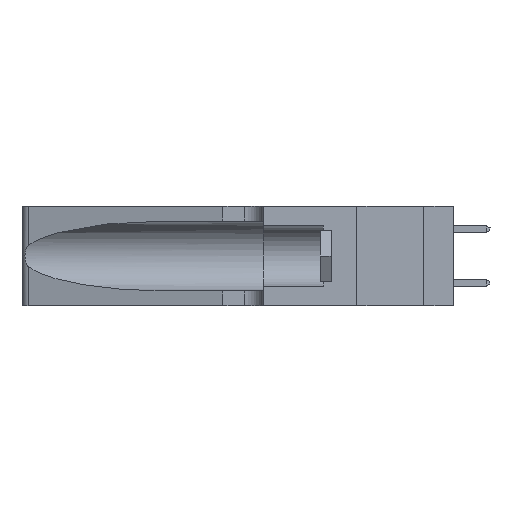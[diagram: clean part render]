
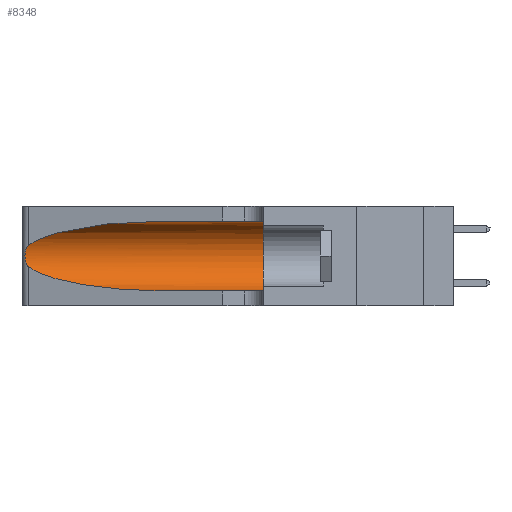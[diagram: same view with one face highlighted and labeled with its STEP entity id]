
A CAD part, left-side view. The second image highlights one B-rep face of the part: STEP entity #8348.
In plain terms, the highlighted cylindrical face has radius 3.308 mm (diameter 6.617 mm), a partial arc.
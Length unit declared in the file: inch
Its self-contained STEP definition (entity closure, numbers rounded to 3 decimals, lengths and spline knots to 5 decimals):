
#110 = VERTEX_POINT ( 'NONE', #4320 ) ;
#845 = CARTESIAN_POINT ( 'NONE',  ( 0.25856, 1.23593, 0.16098 ) ) ;
#872 = B_SPLINE_CURVE_WITH_KNOTS ( 'NONE', 3,
 ( #3177, #21387, #20005, #21594, #1643, #16368, #1378, #8098, #9783, #845, #14072, #4540, #2600, #9413 ),
 .UNSPECIFIED., .F., .F.,
 ( 4, 2, 2, 2, 2, 2, 4 ),
 ( 0., 0.00027, 0.00053, 0.00107, 0.0016, 0.00187, 0.00214 ),
 .UNSPECIFIED. ) ;
#1095 = EDGE_CURVE ( 'NONE', #14580, #16462, #4700, .T. ) ;
#1199 = CARTESIAN_POINT ( 'NONE',  ( 0.1305, 0.72297, 0.31525 ) ) ;
#1378 = CARTESIAN_POINT ( 'NONE',  ( 0.26075, 1.23896, 0.19203 ) ) ;
#1643 = CARTESIAN_POINT ( 'NONE',  ( 0.25854, 1.2359, 0.20912 ) ) ;
#1924 = CARTESIAN_POINT ( 'NONE',  ( 0.1305, 0.35, 0.185 ) ) ;
#2600 = CARTESIAN_POINT ( 'NONE',  ( 0.25555, 1.22993, 0.14849 ) ) ;
#3177 = CARTESIAN_POINT ( 'NONE',  ( 0.25487, 1.22718, 0.22369 ) ) ;
#3914 = ORIENTED_EDGE ( 'NONE', *, *, #4279, .T. ) ;
#4279 = EDGE_CURVE ( 'NONE', #16462, #14871, #872, .T. ) ;
#4320 = CARTESIAN_POINT ( 'NONE',  ( 0.1305, 0.35, 0.05475 ) ) ;
#4540 = CARTESIAN_POINT ( 'NONE',  ( 0.25639, 1.23186, 0.15144 ) ) ;
#4676 = ORIENTED_EDGE ( 'NONE', *, *, #1095, .T. ) ;
#4700 =( BOUNDED_CURVE ( )  B_SPLINE_CURVE ( 3, ( #11744, #16922, #18611, #5336 ),
 .UNSPECIFIED., .F., .T. ) 
 B_SPLINE_CURVE_WITH_KNOTS ( ( 4, 4 ),
 ( 1.5708, 2.84003 ),
 .UNSPECIFIED. ) 
 CURVE ( )  GEOMETRIC_REPRESENTATION_ITEM ( )  RATIONAL_B_SPLINE_CURVE ( ( 1., 0.87, 0.87, 1. ) ) 
 REPRESENTATION_ITEM ( '' )  );
#5022 = DIRECTION ( 'NONE',  ( 0., 1., 0. ) ) ;
#5113 = CARTESIAN_POINT ( 'NONE',  ( 0.1305, 0.72297, 0.05475 ) ) ;
#5336 = CARTESIAN_POINT ( 'NONE',  ( 0.25487, 1.22718, 0.22369 ) ) ;
#5505 = CARTESIAN_POINT ( 'NONE',  ( 0.25487, 1.22718, 0.22369 ) ) ;
#5697 = ORIENTED_EDGE ( 'NONE', *, *, #6693, .F. ) ;
#5938 = CARTESIAN_POINT ( 'NONE',  ( 0.1305, 1.61858, 0.185 ) ) ;
#6017 = VERTEX_POINT ( 'NONE', #18791 ) ;
#6693 = EDGE_CURVE ( 'NONE', #14580, #6017, #19133, .T. ) ;
#6710 = DIRECTION ( 'NONE',  ( 0., 0., 1. ) ) ;
#6713 = AXIS2_PLACEMENT_3D ( 'NONE', #1924, #5022, #6710 ) ;
#6962 =( BOUNDED_CURVE ( )  B_SPLINE_CURVE ( 3, ( #15599, #20641, #7072, #10757 ),
 .UNSPECIFIED., .F., .F. ) 
 B_SPLINE_CURVE_WITH_KNOTS ( ( 4, 4 ),
 ( 3.44316, 4.71239 ),
 .UNSPECIFIED. ) 
 CURVE ( )  GEOMETRIC_REPRESENTATION_ITEM ( )  RATIONAL_B_SPLINE_CURVE ( ( 1., 0.87, 0.87, 1. ) ) 
 REPRESENTATION_ITEM ( '' )  );
#7072 = CARTESIAN_POINT ( 'NONE',  ( 0.18966, 0.96281, 0.05475 ) ) ;
#7772 = CARTESIAN_POINT ( 'NONE',  ( 0.25487, 1.22718, 0.14631 ) ) ;
#8098 = CARTESIAN_POINT ( 'NONE',  ( 0.26075, 1.23896, 0.178 ) ) ;
#8348 = ADVANCED_FACE ( 'NONE', ( #11437 ), #17466, .F. ) ;
#8549 = VECTOR ( 'NONE', #16230, 39.37008 ) ;
#8562 = EDGE_CURVE ( 'NONE', #16965, #110, #13536, .T. ) ;
#9167 = ORIENTED_EDGE ( 'NONE', *, *, #8562, .T. ) ;
#9413 = CARTESIAN_POINT ( 'NONE',  ( 0.25487, 1.22718, 0.14631 ) ) ;
#9783 = CARTESIAN_POINT ( 'NONE',  ( 0.26017, 1.23833, 0.17102 ) ) ;
#9913 = CARTESIAN_POINT ( 'NONE',  ( 0.1305, 1.61858, 0.31525 ) ) ;
#10196 = DIRECTION ( 'NONE',  ( 0., -1., 0. ) ) ;
#10211 = VECTOR ( 'NONE', #10196, 39.37008 ) ;
#10385 = CARTESIAN_POINT ( 'NONE',  ( 0.1305, 1.61858, 0.05475 ) ) ;
#10634 = AXIS2_PLACEMENT_3D ( 'NONE', #5938, #14561, #14402 ) ;
#10757 = CARTESIAN_POINT ( 'NONE',  ( 0.1305, 0.72297, 0.05475 ) ) ;
#11437 = FACE_OUTER_BOUND ( 'NONE', #17543, .T. ) ;
#11640 = ORIENTED_EDGE ( 'NONE', *, *, #15099, .T. ) ;
#11680 = ORIENTED_EDGE ( 'NONE', *, *, #13243, .F. ) ;
#11744 = CARTESIAN_POINT ( 'NONE',  ( 0.1305, 0.72297, 0.31525 ) ) ;
#13243 = EDGE_CURVE ( 'NONE', #6017, #110, #16235, .T. ) ;
#13536 = LINE ( 'NONE', #10385, #8549 ) ;
#14072 = CARTESIAN_POINT ( 'NONE',  ( 0.25789, 1.23486, 0.15765 ) ) ;
#14402 = DIRECTION ( 'NONE',  ( 0., 0., -1. ) ) ;
#14561 = DIRECTION ( 'NONE',  ( 0., -1., 0. ) ) ;
#14580 = VERTEX_POINT ( 'NONE', #1199 ) ;
#14871 = VERTEX_POINT ( 'NONE', #7772 ) ;
#15099 = EDGE_CURVE ( 'NONE', #14871, #16965, #6962, .T. ) ;
#15599 = CARTESIAN_POINT ( 'NONE',  ( 0.25487, 1.22718, 0.14631 ) ) ;
#16230 = DIRECTION ( 'NONE',  ( 0., -1., 0. ) ) ;
#16235 = CIRCLE ( 'NONE', #6713, 0.13025 ) ;
#16368 = CARTESIAN_POINT ( 'NONE',  ( 0.26018, 1.23835, 0.19895 ) ) ;
#16462 = VERTEX_POINT ( 'NONE', #5505 ) ;
#16922 = CARTESIAN_POINT ( 'NONE',  ( 0.18966, 0.96281, 0.31525 ) ) ;
#16965 = VERTEX_POINT ( 'NONE', #5113 ) ;
#17466 = CYLINDRICAL_SURFACE ( 'NONE', #10634, 0.13025 ) ;
#17543 = EDGE_LOOP ( 'NONE', ( #4676, #3914, #11640, #9167, #11680, #5697 ) ) ;
#18611 = CARTESIAN_POINT ( 'NONE',  ( 0.2373, 1.15595, 0.28018 ) ) ;
#18791 = CARTESIAN_POINT ( 'NONE',  ( 0.1305, 0.35, 0.31525 ) ) ;
#19133 = LINE ( 'NONE', #9913, #10211 ) ;
#20005 = CARTESIAN_POINT ( 'NONE',  ( 0.25639, 1.23184, 0.21858 ) ) ;
#20641 = CARTESIAN_POINT ( 'NONE',  ( 0.2373, 1.15595, 0.08982 ) ) ;
#21387 = CARTESIAN_POINT ( 'NONE',  ( 0.25555, 1.22994, 0.2215 ) ) ;
#21594 = CARTESIAN_POINT ( 'NONE',  ( 0.25787, 1.23484, 0.2124 ) ) ;
